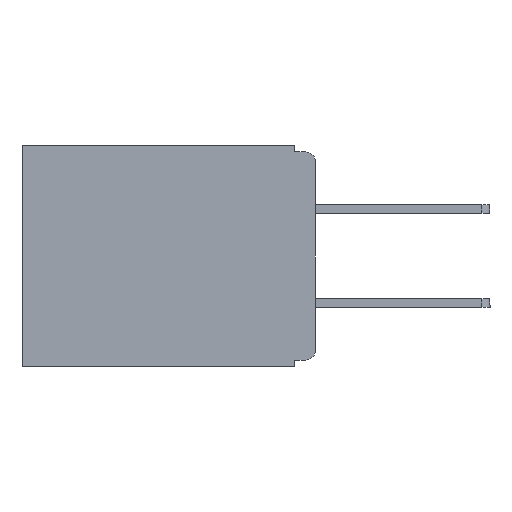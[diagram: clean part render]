
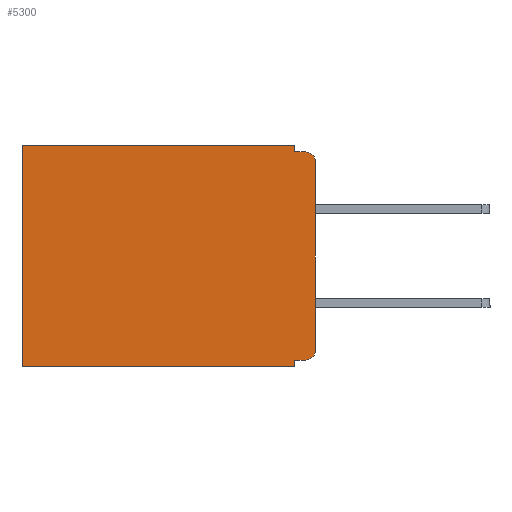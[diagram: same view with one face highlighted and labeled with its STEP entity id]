
A CAD part, left-side view. The second image highlights one B-rep face of the part: STEP entity #5300.
In plain terms, the highlighted planar face has unit normal (-1, 0, 0).
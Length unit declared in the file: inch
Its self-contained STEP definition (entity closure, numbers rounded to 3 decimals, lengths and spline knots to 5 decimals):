
#576 = DIRECTION ( 'NONE',  ( 1., 0., 0. ) ) ;
#696 = AXIS2_PLACEMENT_3D ( 'NONE', #3385, #13129, #11819 ) ;
#719 = DIRECTION ( 'NONE',  ( 0., 0., -1. ) ) ;
#877 = DIRECTION ( 'NONE',  ( 0., 0., -1. ) ) ;
#955 = PLANE ( 'NONE',  #10561 ) ;
#1019 = EDGE_CURVE ( 'NONE', #1720, #2246, #8825, .T. ) ;
#1081 = CARTESIAN_POINT ( 'NONE',  ( 0.3, 0., -0.33 ) ) ;
#1584 = CARTESIAN_POINT ( 'NONE',  ( 0.3, 0.015, -0.01 ) ) ;
#1673 = VECTOR ( 'NONE', #4441, 39.37008 ) ;
#1720 = VERTEX_POINT ( 'NONE', #3341 ) ;
#1865 = VERTEX_POINT ( 'NONE', #14853 ) ;
#2246 = VERTEX_POINT ( 'NONE', #8956 ) ;
#2804 = ORIENTED_EDGE ( 'NONE', *, *, #12404, .F. ) ;
#3341 = CARTESIAN_POINT ( 'NONE',  ( 0.3, 0.015, -0.32 ) ) ;
#3385 = CARTESIAN_POINT ( 'NONE',  ( 0.3, 0.015, -0.305 ) ) ;
#3481 = VERTEX_POINT ( 'NONE', #5163 ) ;
#3582 = DIRECTION ( 'NONE',  ( 0., 1., 0. ) ) ;
#4114 = CARTESIAN_POINT ( 'NONE',  ( 0.3, 0., -0.33 ) ) ;
#4200 = DIRECTION ( 'NONE',  ( 0., -1., 0. ) ) ;
#4241 = DIRECTION ( 'NONE',  ( 0., 0., -1. ) ) ;
#4245 = VERTEX_POINT ( 'NONE', #6777 ) ;
#4418 = EDGE_CURVE ( 'NONE', #1720, #11230, #13798, .T. ) ;
#4441 = DIRECTION ( 'NONE',  ( 0., 0., -1. ) ) ;
#4764 = ORIENTED_EDGE ( 'NONE', *, *, #1019, .F. ) ;
#4788 = LINE ( 'NONE', #11442, #1673 ) ;
#5163 = CARTESIAN_POINT ( 'NONE',  ( 0.3, 0., -0.025 ) ) ;
#5300 = ADVANCED_FACE ( 'NONE', ( #6246 ), #955, .F. ) ;
#6246 = FACE_OUTER_BOUND ( 'NONE', #12060, .T. ) ;
#6427 = DIRECTION ( 'NONE',  ( 0., 1., 0. ) ) ;
#6658 = EDGE_CURVE ( 'NONE', #4245, #6716, #8913, .T. ) ;
#6663 = VECTOR ( 'NONE', #12268, 39.37008 ) ;
#6680 = ORIENTED_EDGE ( 'NONE', *, *, #14228, .F. ) ;
#6716 = VERTEX_POINT ( 'NONE', #14328 ) ;
#6777 = CARTESIAN_POINT ( 'NONE',  ( 0.3, 0.437, 0. ) ) ;
#6992 = EDGE_CURVE ( 'NONE', #3481, #11230, #10000, .T. ) ;
#7286 = CARTESIAN_POINT ( 'NONE',  ( 0.3, 0.437, -0.33 ) ) ;
#7437 = ORIENTED_EDGE ( 'NONE', *, *, #11185, .F. ) ;
#7491 = VERTEX_POINT ( 'NONE', #1584 ) ;
#7705 = DIRECTION ( 'NONE',  ( -1., 0., 0. ) ) ;
#7878 = ORIENTED_EDGE ( 'NONE', *, *, #4418, .T. ) ;
#8825 = LINE ( 'NONE', #10678, #14956 ) ;
#8913 = LINE ( 'NONE', #7286, #12719 ) ;
#8956 = CARTESIAN_POINT ( 'NONE',  ( 0.3, 0.031, -0.32 ) ) ;
#8969 = CARTESIAN_POINT ( 'NONE',  ( 0.3, 0., -0.305 ) ) ;
#9072 = VERTEX_POINT ( 'NONE', #14081 ) ;
#9324 = VECTOR ( 'NONE', #10092, 39.37008 ) ;
#9417 = CARTESIAN_POINT ( 'NONE',  ( 0.3, 0., -0.33 ) ) ;
#9485 = CARTESIAN_POINT ( 'NONE',  ( 0.3, 0., 0. ) ) ;
#9527 = DIRECTION ( 'NONE',  ( 0., 0., -1. ) ) ;
#9586 = VECTOR ( 'NONE', #4200, 39.37008 ) ;
#9734 = ORIENTED_EDGE ( 'NONE', *, *, #11953, .F. ) ;
#9740 = LINE ( 'NONE', #4114, #6663 ) ;
#9904 = EDGE_CURVE ( 'NONE', #3481, #7491, #11564, .T. ) ;
#10000 = LINE ( 'NONE', #9417, #13055 ) ;
#10092 = DIRECTION ( 'NONE',  ( 0., 0., -1. ) ) ;
#10286 = VERTEX_POINT ( 'NONE', #14102 ) ;
#10303 = ORIENTED_EDGE ( 'NONE', *, *, #9904, .T. ) ;
#10472 = ORIENTED_EDGE ( 'NONE', *, *, #6658, .T. ) ;
#10561 = AXIS2_PLACEMENT_3D ( 'NONE', #1081, #576, #877 ) ;
#10678 = CARTESIAN_POINT ( 'NONE',  ( 0.3, 0., -0.32 ) ) ;
#10832 = VECTOR ( 'NONE', #3582, 39.37008 ) ;
#11185 = EDGE_CURVE ( 'NONE', #10286, #7491, #12651, .T. ) ;
#11196 = LINE ( 'NONE', #9485, #10832 ) ;
#11230 = VERTEX_POINT ( 'NONE', #8969 ) ;
#11293 = ORIENTED_EDGE ( 'NONE', *, *, #6992, .F. ) ;
#11442 = CARTESIAN_POINT ( 'NONE',  ( 0.3, 0.031, -0.33 ) ) ;
#11564 = CIRCLE ( 'NONE', #11988, 0.015 ) ;
#11819 = DIRECTION ( 'NONE',  ( 0., 0., -1. ) ) ;
#11953 = EDGE_CURVE ( 'NONE', #2246, #1865, #4788, .T. ) ;
#11988 = AXIS2_PLACEMENT_3D ( 'NONE', #14615, #7705, #719 ) ;
#12060 = EDGE_LOOP ( 'NONE', ( #11293, #10303, #7437, #6680, #12329, #10472, #2804, #9734, #4764, #7878 ) ) ;
#12268 = DIRECTION ( 'NONE',  ( 0., 1., 0. ) ) ;
#12329 = ORIENTED_EDGE ( 'NONE', *, *, #12776, .T. ) ;
#12392 = LINE ( 'NONE', #13568, #9324 ) ;
#12404 = EDGE_CURVE ( 'NONE', #1865, #6716, #9740, .T. ) ;
#12651 = LINE ( 'NONE', #14616, #9586 ) ;
#12719 = VECTOR ( 'NONE', #4241, 39.37008 ) ;
#12776 = EDGE_CURVE ( 'NONE', #9072, #4245, #11196, .T. ) ;
#13055 = VECTOR ( 'NONE', #9527, 39.37008 ) ;
#13129 = DIRECTION ( 'NONE',  ( -1., 0., 0. ) ) ;
#13568 = CARTESIAN_POINT ( 'NONE',  ( 0.3, 0.031, 0. ) ) ;
#13798 = CIRCLE ( 'NONE', #696, 0.015 ) ;
#14081 = CARTESIAN_POINT ( 'NONE',  ( 0.3, 0.031, 0. ) ) ;
#14102 = CARTESIAN_POINT ( 'NONE',  ( 0.3, 0.031, -0.01 ) ) ;
#14228 = EDGE_CURVE ( 'NONE', #9072, #10286, #12392, .T. ) ;
#14328 = CARTESIAN_POINT ( 'NONE',  ( 0.3, 0.437, -0.33 ) ) ;
#14615 = CARTESIAN_POINT ( 'NONE',  ( 0.3, 0.015, -0.025 ) ) ;
#14616 = CARTESIAN_POINT ( 'NONE',  ( 0.3, 0., -0.01 ) ) ;
#14853 = CARTESIAN_POINT ( 'NONE',  ( 0.3, 0.031, -0.33 ) ) ;
#14956 = VECTOR ( 'NONE', #6427, 39.37008 ) ;
